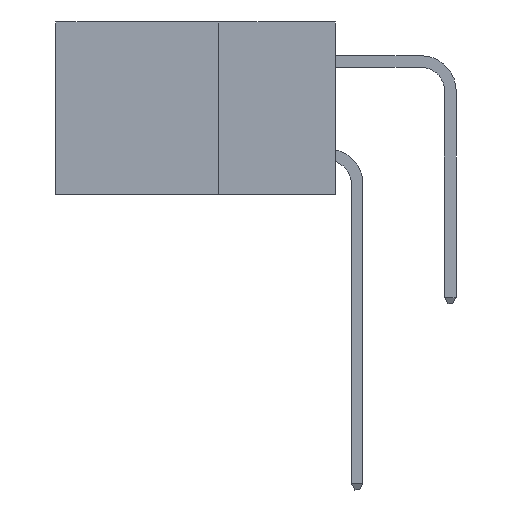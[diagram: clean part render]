
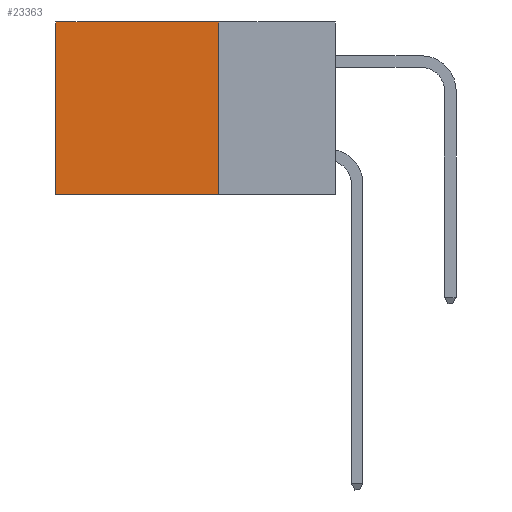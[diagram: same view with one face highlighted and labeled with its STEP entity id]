
A CAD part, left-side view. The second image highlights one B-rep face of the part: STEP entity #23363.
In plain terms, the highlighted planar face has unit normal (-1, 0, 0).
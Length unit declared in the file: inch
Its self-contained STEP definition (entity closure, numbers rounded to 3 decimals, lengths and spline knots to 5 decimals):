
#1280 = FACE_OUTER_BOUND ( 'NONE', #6445, .T. ) ;
#2607 = VERTEX_POINT ( 'NONE', #10903 ) ;
#3791 = EDGE_CURVE ( 'NONE', #11968, #26797, #15466, .T. ) ;
#4996 = CARTESIAN_POINT ( 'NONE',  ( 0.2875, 0.6, 0. ) ) ;
#5315 = CARTESIAN_POINT ( 'NONE',  ( 0.2875, 0.25, -0.37 ) ) ;
#5944 = VECTOR ( 'NONE', #28647, 39.37008 ) ;
#6445 = EDGE_LOOP ( 'NONE', ( #16261, #11253, #8612, #18546 ) ) ;
#6933 = DIRECTION ( 'NONE',  ( 0., 1., 0. ) ) ;
#8612 = ORIENTED_EDGE ( 'NONE', *, *, #21935, .F. ) ;
#10224 = LINE ( 'NONE', #12547, #30990 ) ;
#10903 = CARTESIAN_POINT ( 'NONE',  ( 0.2875, 0.6, -0.37 ) ) ;
#11253 = ORIENTED_EDGE ( 'NONE', *, *, #14759, .F. ) ;
#11968 = VERTEX_POINT ( 'NONE', #23242 ) ;
#12547 = CARTESIAN_POINT ( 'NONE',  ( 0.2875, 0.25, 0. ) ) ;
#13122 = AXIS2_PLACEMENT_3D ( 'NONE', #36200, #36776, #19185 ) ;
#14759 = EDGE_CURVE ( 'NONE', #29705, #2607, #22060, .T. ) ;
#15466 = LINE ( 'NONE', #15848, #36901 ) ;
#15848 = CARTESIAN_POINT ( 'NONE',  ( 0.2875, 0.25, 0. ) ) ;
#16261 = ORIENTED_EDGE ( 'NONE', *, *, #34540, .T. ) ;
#18546 = ORIENTED_EDGE ( 'NONE', *, *, #3791, .T. ) ;
#18802 = DIRECTION ( 'NONE',  ( 0., 0., -1. ) ) ;
#19185 = DIRECTION ( 'NONE',  ( 0., 0., -1. ) ) ;
#19768 = LINE ( 'NONE', #4996, #5944 ) ;
#20767 = CARTESIAN_POINT ( 'NONE',  ( 0.2875, 0.6, 0. ) ) ;
#21682 = CARTESIAN_POINT ( 'NONE',  ( 0.2875, 0.25, -0.37 ) ) ;
#21935 = EDGE_CURVE ( 'NONE', #11968, #29705, #10224, .T. ) ;
#22060 = LINE ( 'NONE', #21682, #31862 ) ;
#23242 = CARTESIAN_POINT ( 'NONE',  ( 0.2875, 0.25, 0. ) ) ;
#23363 = ADVANCED_FACE ( 'NONE', ( #1280 ), #24383, .F. ) ;
#24383 = PLANE ( 'NONE',  #13122 ) ;
#26797 = VERTEX_POINT ( 'NONE', #20767 ) ;
#28647 = DIRECTION ( 'NONE',  ( 0., 0., -1. ) ) ;
#29705 = VERTEX_POINT ( 'NONE', #5315 ) ;
#30990 = VECTOR ( 'NONE', #18802, 39.37008 ) ;
#31862 = VECTOR ( 'NONE', #6933, 39.37008 ) ;
#33096 = DIRECTION ( 'NONE',  ( 0., 1., 0. ) ) ;
#34540 = EDGE_CURVE ( 'NONE', #26797, #2607, #19768, .T. ) ;
#36200 = CARTESIAN_POINT ( 'NONE',  ( 0.2875, 0.25, 0. ) ) ;
#36776 = DIRECTION ( 'NONE',  ( 1., 0., 0. ) ) ;
#36901 = VECTOR ( 'NONE', #33096, 39.37008 ) ;
